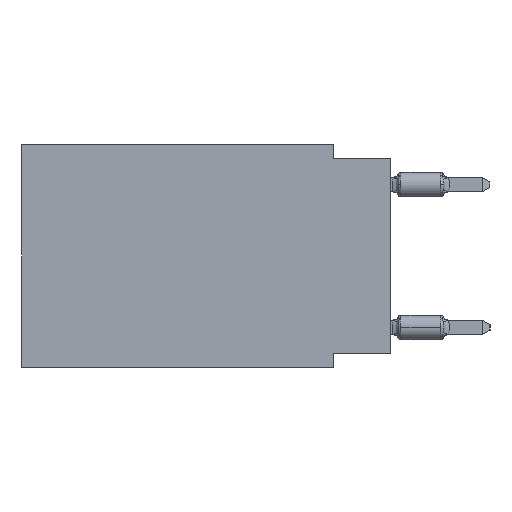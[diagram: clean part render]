
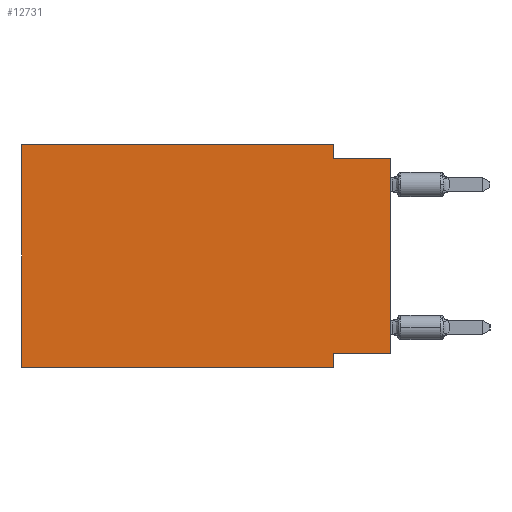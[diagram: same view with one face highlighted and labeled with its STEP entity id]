
A CAD part, left-side view. The second image highlights one B-rep face of the part: STEP entity #12731.
In plain terms, the highlighted planar face has unit normal (-1, 0, 0).
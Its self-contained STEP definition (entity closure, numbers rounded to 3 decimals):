
#20 = DIRECTION ( 'NONE',  ( 0., 0., 1. ) ) ;
#139 = LINE ( 'NONE', #19686, #9564 ) ;
#272 = EDGE_CURVE ( 'NONE', #13991, #13721, #15412, .T. ) ;
#352 = DIRECTION ( 'NONE',  ( 0., 1., 0. ) ) ;
#590 = CARTESIAN_POINT ( 'NONE',  ( 0., 0., -0.635 ) ) ;
#748 = EDGE_CURVE ( 'NONE', #25952, #9928, #139, .T. ) ;
#979 = VECTOR ( 'NONE', #20, 1000. ) ;
#1424 = CARTESIAN_POINT ( 'NONE',  ( 0., 2.54, -9.271 ) ) ;
#1445 = CARTESIAN_POINT ( 'NONE',  ( 0., 2.54, 0. ) ) ;
#1484 = CARTESIAN_POINT ( 'NONE',  ( 0., 0., -9.271 ) ) ;
#1809 = ORIENTED_EDGE ( 'NONE', *, *, #24165, .F. ) ;
#1902 = CARTESIAN_POINT ( 'NONE',  ( 0., 16.383, 0. ) ) ;
#2436 = EDGE_LOOP ( 'NONE', ( #6926, #8126, #28204, #16461, #14043, #8927, #26251, #1809 ) ) ;
#2567 = PLANE ( 'NONE',  #19780 ) ;
#3281 = VECTOR ( 'NONE', #10200, 1000. ) ;
#4136 = VERTEX_POINT ( 'NONE', #22281 ) ;
#4857 = DIRECTION ( 'NONE',  ( 0., 0., -1. ) ) ;
#5029 = CARTESIAN_POINT ( 'NONE',  ( 0., 16.383, 0. ) ) ;
#6101 = DIRECTION ( 'NONE',  ( 0., -1., 0. ) ) ;
#6456 = VERTEX_POINT ( 'NONE', #15057 ) ;
#6627 = EDGE_CURVE ( 'NONE', #23741, #4136, #7163, .T. ) ;
#6926 = ORIENTED_EDGE ( 'NONE', *, *, #748, .T. ) ;
#7163 = LINE ( 'NONE', #13763, #19591 ) ;
#7695 = LINE ( 'NONE', #25211, #14586 ) ;
#7976 = DIRECTION ( 'NONE',  ( 0., -1., 0. ) ) ;
#8126 = ORIENTED_EDGE ( 'NONE', *, *, #9240, .F. ) ;
#8927 = ORIENTED_EDGE ( 'NONE', *, *, #13371, .T. ) ;
#9240 = EDGE_CURVE ( 'NONE', #11919, #9928, #7695, .T. ) ;
#9564 = VECTOR ( 'NONE', #20101, 1000. ) ;
#9928 = VERTEX_POINT ( 'NONE', #590 ) ;
#10200 = DIRECTION ( 'NONE',  ( 0., 0., -1. ) ) ;
#11077 = LINE ( 'NONE', #1902, #979 ) ;
#11919 = VERTEX_POINT ( 'NONE', #18701 ) ;
#12094 = EDGE_CURVE ( 'NONE', #6456, #23741, #11077, .T. ) ;
#12569 = CARTESIAN_POINT ( 'NONE',  ( 0., 16.383, -9.906 ) ) ;
#12731 = ADVANCED_FACE ( 'NONE', ( #22229 ), #2567, .F. ) ;
#13371 = EDGE_CURVE ( 'NONE', #6456, #13721, #19025, .T. ) ;
#13721 = VERTEX_POINT ( 'NONE', #15332 ) ;
#13763 = CARTESIAN_POINT ( 'NONE',  ( 0., 16.383, 0. ) ) ;
#13986 = LINE ( 'NONE', #22763, #25904 ) ;
#13991 = VERTEX_POINT ( 'NONE', #1424 ) ;
#14043 = ORIENTED_EDGE ( 'NONE', *, *, #12094, .F. ) ;
#14586 = VECTOR ( 'NONE', #7976, 1000. ) ;
#15057 = CARTESIAN_POINT ( 'NONE',  ( 0., 16.383, -9.906 ) ) ;
#15332 = CARTESIAN_POINT ( 'NONE',  ( 0., 2.54, -9.906 ) ) ;
#15412 = LINE ( 'NONE', #21886, #25132 ) ;
#16461 = ORIENTED_EDGE ( 'NONE', *, *, #6627, .F. ) ;
#16615 = DIRECTION ( 'NONE',  ( 0., -1., 0. ) ) ;
#16769 = LINE ( 'NONE', #1445, #3281 ) ;
#17511 = EDGE_CURVE ( 'NONE', #4136, #11919, #16769, .T. ) ;
#18701 = CARTESIAN_POINT ( 'NONE',  ( 0., 2.54, -0.635 ) ) ;
#19025 = LINE ( 'NONE', #12569, #23428 ) ;
#19591 = VECTOR ( 'NONE', #16615, 1000. ) ;
#19686 = CARTESIAN_POINT ( 'NONE',  ( 0., 0., 0. ) ) ;
#19780 = AXIS2_PLACEMENT_3D ( 'NONE', #24528, #22678, #4857 ) ;
#20101 = DIRECTION ( 'NONE',  ( 0., 0., 1. ) ) ;
#21886 = CARTESIAN_POINT ( 'NONE',  ( 0., 2.54, -9.906 ) ) ;
#22229 = FACE_OUTER_BOUND ( 'NONE', #2436, .T. ) ;
#22281 = CARTESIAN_POINT ( 'NONE',  ( 0., 2.54, 0. ) ) ;
#22678 = DIRECTION ( 'NONE',  ( 1., 0., 0. ) ) ;
#22763 = CARTESIAN_POINT ( 'NONE',  ( 0., 0., -9.271 ) ) ;
#23428 = VECTOR ( 'NONE', #6101, 1000. ) ;
#23741 = VERTEX_POINT ( 'NONE', #5029 ) ;
#24165 = EDGE_CURVE ( 'NONE', #25952, #13991, #13986, .T. ) ;
#24528 = CARTESIAN_POINT ( 'NONE',  ( 0., 16.383, 0. ) ) ;
#25132 = VECTOR ( 'NONE', #26345, 1000. ) ;
#25211 = CARTESIAN_POINT ( 'NONE',  ( 0., 0., -0.635 ) ) ;
#25904 = VECTOR ( 'NONE', #352, 1000. ) ;
#25952 = VERTEX_POINT ( 'NONE', #1484 ) ;
#26251 = ORIENTED_EDGE ( 'NONE', *, *, #272, .F. ) ;
#26345 = DIRECTION ( 'NONE',  ( 0., 0., -1. ) ) ;
#28204 = ORIENTED_EDGE ( 'NONE', *, *, #17511, .F. ) ;
